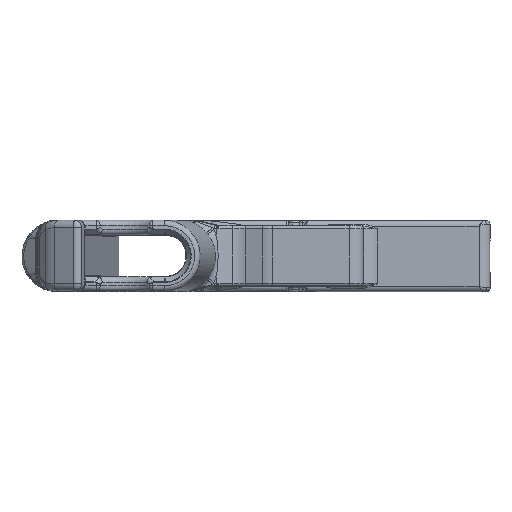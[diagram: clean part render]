
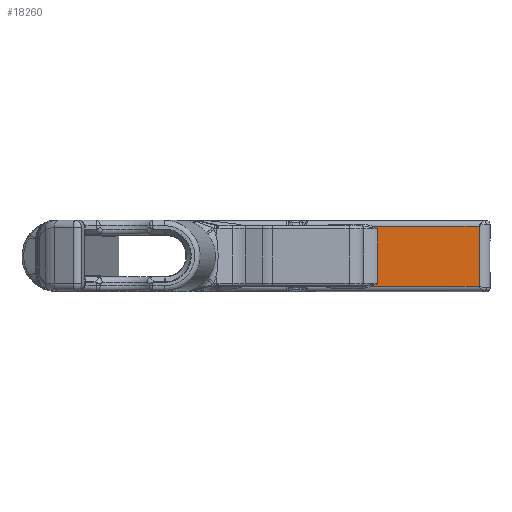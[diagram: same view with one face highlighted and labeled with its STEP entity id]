
A CAD part, top view. The second image highlights one B-rep face of the part: STEP entity #18260.
In plain terms, the highlighted planar face has unit normal (0, 0, 1).
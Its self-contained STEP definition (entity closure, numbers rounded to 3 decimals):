
#750=B_SPLINE_CURVE_WITH_KNOTS('',3,(#35994,#35995,#35996,#35997,#35998,
#35999),.UNSPECIFIED.,.F.,.F.,(4,2,4),(-0.155,0.,0.001),
 .UNSPECIFIED.);
#760=B_SPLINE_CURVE_WITH_KNOTS('',3,(#36144,#36145,#36146,#36147,#36148,
#36149),.UNSPECIFIED.,.F.,.F.,(4,2,4),(-0.156,-0.155,
0.),.UNSPECIFIED.);
#1652=PLANE('',#19927);
#2295=FACE_OUTER_BOUND('',#3538,.T.);
#3538=EDGE_LOOP('',(#14069,#14070,#14071,#14072,#14073,#14074));
#4669=LINE('',#36138,#5493);
#4670=LINE('',#36140,#5494);
#4671=LINE('',#36142,#5495);
#4672=LINE('',#36150,#5496);
#5493=VECTOR('',#23377,10.);
#5494=VECTOR('',#23378,10.);
#5495=VECTOR('',#23379,10.);
#5496=VECTOR('',#23380,10.);
#7915=VERTEX_POINT('',#35992);
#7916=VERTEX_POINT('',#35993);
#7950=VERTEX_POINT('',#36137);
#7951=VERTEX_POINT('',#36139);
#7952=VERTEX_POINT('',#36141);
#7953=VERTEX_POINT('',#36143);
#10081=EDGE_CURVE('',#7915,#7916,#750,.T.);
#10121=EDGE_CURVE('',#7950,#7915,#4669,.T.);
#10122=EDGE_CURVE('',#7951,#7950,#4670,.T.);
#10123=EDGE_CURVE('',#7952,#7951,#4671,.T.);
#10124=EDGE_CURVE('',#7953,#7952,#760,.T.);
#10125=EDGE_CURVE('',#7916,#7953,#4672,.T.);
#14069=ORIENTED_EDGE('',*,*,#10081,.F.);
#14070=ORIENTED_EDGE('',*,*,#10121,.F.);
#14071=ORIENTED_EDGE('',*,*,#10122,.F.);
#14072=ORIENTED_EDGE('',*,*,#10123,.F.);
#14073=ORIENTED_EDGE('',*,*,#10124,.F.);
#14074=ORIENTED_EDGE('',*,*,#10125,.F.);
#18260=ADVANCED_FACE('',(#2295),#1652,.F.);
#19927=AXIS2_PLACEMENT_3D('',#36136,#23375,#23376);
#23375=DIRECTION('center_axis',(0.,0.,-1.));
#23376=DIRECTION('ref_axis',(-1.,0.,0.));
#23377=DIRECTION('',(-1.,0.,0.));
#23378=DIRECTION('',(0.,-1.,0.));
#23379=DIRECTION('',(1.,0.,0.));
#23380=DIRECTION('',(0.,1.,0.));
#35992=CARTESIAN_POINT('',(30.672,-8.25,-14.25));
#35993=CARTESIAN_POINT('',(32.04,-7.5,-14.25));
#35994=CARTESIAN_POINT('Ctrl Pts',(30.672,-8.25,-14.25));
#35995=CARTESIAN_POINT('Ctrl Pts',(31.133,-8.016,-14.25));
#35996=CARTESIAN_POINT('Ctrl Pts',(31.582,-7.76,-14.25));
#35997=CARTESIAN_POINT('Ctrl Pts',(32.034,-7.503,-14.25));
#35998=CARTESIAN_POINT('Ctrl Pts',(32.037,-7.502,-14.25));
#35999=CARTESIAN_POINT('Ctrl Pts',(32.04,-7.5,-14.25));
#36136=CARTESIAN_POINT('Origin',(15.5,0.,-14.25));
#36137=CARTESIAN_POINT('',(60.,-8.25,-14.25));
#36138=CARTESIAN_POINT('',(7.087,-8.25,-14.25));
#36139=CARTESIAN_POINT('',(60.,8.25,-14.25));
#36140=CARTESIAN_POINT('',(60.,0.,-14.25));
#36141=CARTESIAN_POINT('',(30.672,8.25,-14.25));
#36142=CARTESIAN_POINT('',(7.087,8.25,-14.25));
#36143=CARTESIAN_POINT('',(32.04,7.5,-14.25));
#36144=CARTESIAN_POINT('Ctrl Pts',(32.04,7.5,-14.25));
#36145=CARTESIAN_POINT('Ctrl Pts',(32.037,7.502,-14.25));
#36146=CARTESIAN_POINT('Ctrl Pts',(32.034,7.503,-14.25));
#36147=CARTESIAN_POINT('Ctrl Pts',(31.582,7.76,-14.25));
#36148=CARTESIAN_POINT('Ctrl Pts',(31.133,8.016,-14.25));
#36149=CARTESIAN_POINT('Ctrl Pts',(30.672,8.25,-14.25));
#36150=CARTESIAN_POINT('',(32.04,0.,-14.25));
